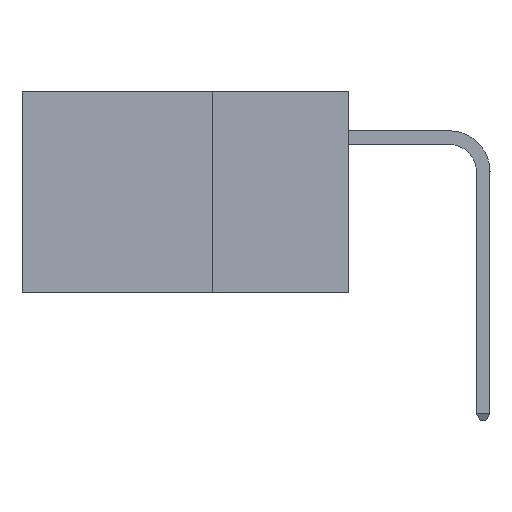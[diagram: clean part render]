
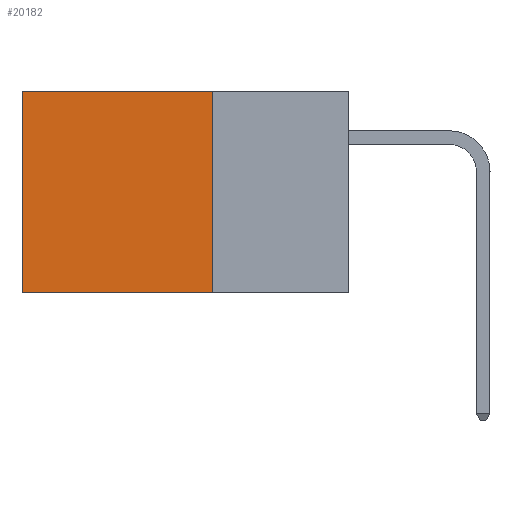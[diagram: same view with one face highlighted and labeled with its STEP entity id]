
A CAD part, left-side view. The second image highlights one B-rep face of the part: STEP entity #20182.
In plain terms, the highlighted planar face has unit normal (-1, 0, 0).
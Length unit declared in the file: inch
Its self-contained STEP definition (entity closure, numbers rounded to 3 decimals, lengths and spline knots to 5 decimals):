
#873 = ORIENTED_EDGE ( 'NONE', *, *, #14149, .T. ) ;
#2100 = DIRECTION ( 'NONE',  ( 0., 0., -1. ) ) ;
#2450 = CARTESIAN_POINT ( 'NONE',  ( 0.2875, 0.25, -0.37 ) ) ;
#2977 = DIRECTION ( 'NONE',  ( 0., 0., -1. ) ) ;
#3599 = VECTOR ( 'NONE', #2100, 39.37008 ) ;
#4012 = VECTOR ( 'NONE', #18888, 39.37008 ) ;
#4611 = EDGE_CURVE ( 'NONE', #34077, #11629, #6741, .T. ) ;
#4986 = CARTESIAN_POINT ( 'NONE',  ( 0.2875, 0.6, 0. ) ) ;
#5105 = EDGE_CURVE ( 'NONE', #6331, #32215, #11595, .T. ) ;
#6037 = AXIS2_PLACEMENT_3D ( 'NONE', #10355, #27069, #10483 ) ;
#6331 = VERTEX_POINT ( 'NONE', #21174 ) ;
#6741 = LINE ( 'NONE', #30334, #28065 ) ;
#7065 = EDGE_LOOP ( 'NONE', ( #873, #15146, #23801, #15975 ) ) ;
#7626 = PLANE ( 'NONE',  #6037 ) ;
#9813 = VECTOR ( 'NONE', #2977, 39.37008 ) ;
#10355 = CARTESIAN_POINT ( 'NONE',  ( 0.2875, 0.25, 0. ) ) ;
#10483 = DIRECTION ( 'NONE',  ( 0., 0., -1. ) ) ;
#11595 = LINE ( 'NONE', #13280, #4012 ) ;
#11629 = VERTEX_POINT ( 'NONE', #23473 ) ;
#12456 = EDGE_CURVE ( 'NONE', #6331, #34077, #31830, .T. ) ;
#13280 = CARTESIAN_POINT ( 'NONE',  ( 0.2875, 0.25, 0. ) ) ;
#14149 = EDGE_CURVE ( 'NONE', #32215, #11629, #18652, .T. ) ;
#14311 = CARTESIAN_POINT ( 'NONE',  ( 0.2875, 0.6, 0. ) ) ;
#15146 = ORIENTED_EDGE ( 'NONE', *, *, #4611, .F. ) ;
#15975 = ORIENTED_EDGE ( 'NONE', *, *, #5105, .T. ) ;
#17130 = CARTESIAN_POINT ( 'NONE',  ( 0.2875, 0.25, 0. ) ) ;
#18652 = LINE ( 'NONE', #4986, #3599 ) ;
#18888 = DIRECTION ( 'NONE',  ( 0., 1., 0. ) ) ;
#19530 = DIRECTION ( 'NONE',  ( 0., 1., 0. ) ) ;
#20182 = ADVANCED_FACE ( 'NONE', ( #34229 ), #7626, .F. ) ;
#21174 = CARTESIAN_POINT ( 'NONE',  ( 0.2875, 0.25, 0. ) ) ;
#23473 = CARTESIAN_POINT ( 'NONE',  ( 0.2875, 0.6, -0.37 ) ) ;
#23801 = ORIENTED_EDGE ( 'NONE', *, *, #12456, .F. ) ;
#27069 = DIRECTION ( 'NONE',  ( 1., 0., 0. ) ) ;
#28065 = VECTOR ( 'NONE', #19530, 39.37008 ) ;
#30334 = CARTESIAN_POINT ( 'NONE',  ( 0.2875, 0.25, -0.37 ) ) ;
#31830 = LINE ( 'NONE', #17130, #9813 ) ;
#32215 = VERTEX_POINT ( 'NONE', #14311 ) ;
#34077 = VERTEX_POINT ( 'NONE', #2450 ) ;
#34229 = FACE_OUTER_BOUND ( 'NONE', #7065, .T. ) ;
